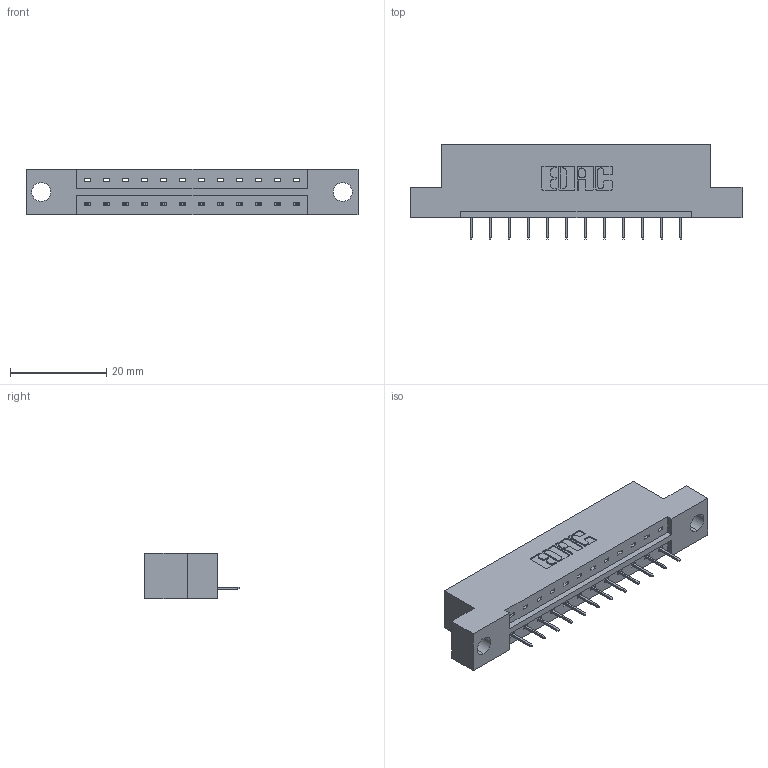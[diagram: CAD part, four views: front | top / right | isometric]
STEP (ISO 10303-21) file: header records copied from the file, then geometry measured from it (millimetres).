
FILE_DESCRIPTION (( 'STEP AP203' ), '1' );
FILE_NAME ('833-012-524-104.STEP', '2020-05-30T21:23:38', ( '' ), ( '' ), 'SwSTEP 2.0', 'SolidWorks 2020', '' );
FILE_SCHEMA (( 'CONFIG_CONTROL_DESIGN' ));
Length unit declared in the file: inch
Products named in the file (3): 345-292-001_345-293-124; 833 Part_Flush - .156 Dia - TH; 833-012-524-104
Assembly tree (13 placements, depth 2):
  833-012-524-104
    833 Part_Flush - .156 Dia - TH
    345-292-001_345-293-124  x12
Bounding box: 69.09 x 19.69 x 9.4 mm (x, y, z)
Volume: 6558.9 mm3; surface area: 6532.7 mm2
Topology: 13 solids, 13 shells, 858 faces, 2471 edges, 1598 vertices
Faces by surface type: plane 646, cylinder 212
Entity records: 11293 total; most frequent: CARTESIAN_POINT 1958, ORIENTED_EDGE 1906, DIRECTION 1713, EDGE_CURVE 953, LINE 829, VECTOR 829, VERTEX_POINT 630, AXIS2_PLACEMENT_3D 442
